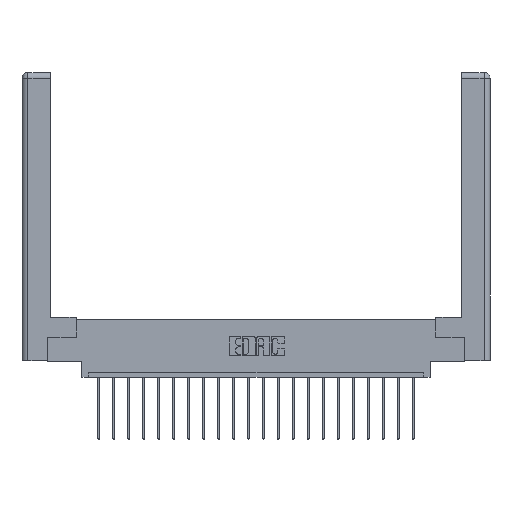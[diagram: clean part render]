
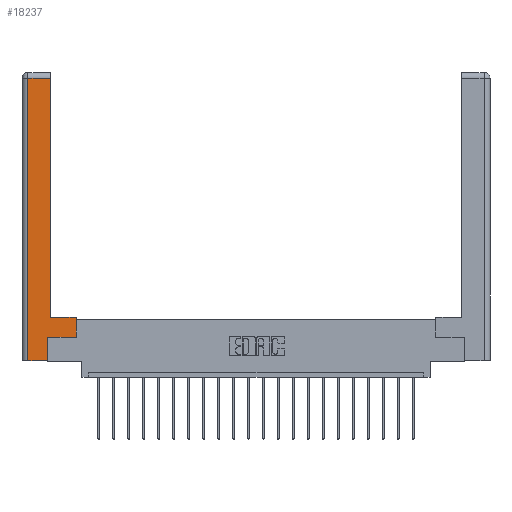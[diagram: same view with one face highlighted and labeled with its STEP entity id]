
A CAD part, top view. The second image highlights one B-rep face of the part: STEP entity #18237.
In plain terms, the highlighted planar face has unit normal (0, 0, 1).
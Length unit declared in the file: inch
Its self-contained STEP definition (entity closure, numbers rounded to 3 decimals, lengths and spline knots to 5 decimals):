
#123 = ORIENTED_EDGE ( 'NONE', *, *, #9968, .T. ) ;
#408 = DIRECTION ( 'NONE',  ( 1., 0., 0. ) ) ;
#514 = ORIENTED_EDGE ( 'NONE', *, *, #17847, .T. ) ;
#659 = VERTEX_POINT ( 'NONE', #21125 ) ;
#902 = ORIENTED_EDGE ( 'NONE', *, *, #16288, .T. ) ;
#1012 = VERTEX_POINT ( 'NONE', #8918 ) ;
#1280 = VECTOR ( 'NONE', #16878, 39.37008 ) ;
#1585 = CARTESIAN_POINT ( 'NONE',  ( 0.0615, 2.94, 0. ) ) ;
#1903 = LINE ( 'NONE', #21490, #8212 ) ;
#2290 = CARTESIAN_POINT ( 'NONE',  ( 0.0615, 2.94, 0. ) ) ;
#2301 = CARTESIAN_POINT ( 'NONE',  ( 0., 0., 0. ) ) ;
#2375 = ORIENTED_EDGE ( 'NONE', *, *, #11505, .T. ) ;
#2445 = ORIENTED_EDGE ( 'NONE', *, *, #6654, .T. ) ;
#2831 = CARTESIAN_POINT ( 'NONE',  ( 0.295, 0.45, 0. ) ) ;
#3074 = DIRECTION ( 'NONE',  ( 0., -1., 0. ) ) ;
#3162 = VERTEX_POINT ( 'NONE', #2831 ) ;
#3676 = VERTEX_POINT ( 'NONE', #1585 ) ;
#3696 = CARTESIAN_POINT ( 'NONE',  ( 0.565, 0.45, 0. ) ) ;
#3892 = VECTOR ( 'NONE', #10589, 39.37008 ) ;
#5469 = LINE ( 'NONE', #3696, #1280 ) ;
#5729 = FACE_OUTER_BOUND ( 'NONE', #6159, .T. ) ;
#5975 = EDGE_CURVE ( 'NONE', #6447, #12346, #18873, .T. ) ;
#6159 = EDGE_LOOP ( 'NONE', ( #123, #2375, #902, #514, #2445, #20924, #20178, #9627 ) ) ;
#6378 = DIRECTION ( 'NONE',  ( -1., 0., 0. ) ) ;
#6447 = VERTEX_POINT ( 'NONE', #14517 ) ;
#6654 = EDGE_CURVE ( 'NONE', #659, #6447, #13541, .T. ) ;
#7048 = DIRECTION ( 'NONE',  ( 0., 1., 0. ) ) ;
#7058 = CARTESIAN_POINT ( 'NONE',  ( 0.565, 0.245, 0. ) ) ;
#7818 = LINE ( 'NONE', #17628, #10714 ) ;
#7833 = LINE ( 'NONE', #2290, #3892 ) ;
#7867 = VECTOR ( 'NONE', #21477, 39.37008 ) ;
#8212 = VECTOR ( 'NONE', #3074, 39.37008 ) ;
#8342 = VECTOR ( 'NONE', #408, 39.37008 ) ;
#8636 = CARTESIAN_POINT ( 'NONE',  ( 0.295, 2.94, 0. ) ) ;
#8918 = CARTESIAN_POINT ( 'NONE',  ( 0.0615, 0., 0. ) ) ;
#9627 = ORIENTED_EDGE ( 'NONE', *, *, #21451, .T. ) ;
#9968 = EDGE_CURVE ( 'NONE', #3162, #17241, #13345, .T. ) ;
#10589 = DIRECTION ( 'NONE',  ( -1., 0., 0. ) ) ;
#10714 = VECTOR ( 'NONE', #6378, 39.37008 ) ;
#10739 = CARTESIAN_POINT ( 'NONE',  ( 0.295, 3., 0. ) ) ;
#10893 = DIRECTION ( 'NONE',  ( -1., 0., 0. ) ) ;
#11313 = EDGE_CURVE ( 'NONE', #12346, #21047, #5469, .T. ) ;
#11505 = EDGE_CURVE ( 'NONE', #17241, #3676, #7833, .T. ) ;
#12336 = PLANE ( 'NONE',  #20123 ) ;
#12346 = VERTEX_POINT ( 'NONE', #17895 ) ;
#13345 = LINE ( 'NONE', #10739, #17835 ) ;
#13541 = LINE ( 'NONE', #14880, #15376 ) ;
#14517 = CARTESIAN_POINT ( 'NONE',  ( 0.265, 0.245, 0. ) ) ;
#14880 = CARTESIAN_POINT ( 'NONE',  ( 0.265, 0.245, 0. ) ) ;
#15376 = VECTOR ( 'NONE', #16559, 39.37008 ) ;
#16288 = EDGE_CURVE ( 'NONE', #3676, #1012, #1903, .T. ) ;
#16559 = DIRECTION ( 'NONE',  ( 0., 1., 0. ) ) ;
#16657 = CARTESIAN_POINT ( 'NONE',  ( 0.565, 0.45, 0. ) ) ;
#16878 = DIRECTION ( 'NONE',  ( 0., 1., 0. ) ) ;
#17241 = VERTEX_POINT ( 'NONE', #8636 ) ;
#17628 = CARTESIAN_POINT ( 'NONE',  ( 0.295, 0.45, 0. ) ) ;
#17835 = VECTOR ( 'NONE', #7048, 39.37008 ) ;
#17847 = EDGE_CURVE ( 'NONE', #1012, #659, #21273, .T. ) ;
#17895 = CARTESIAN_POINT ( 'NONE',  ( 0.565, 0.245, 0. ) ) ;
#18237 = ADVANCED_FACE ( 'NONE', ( #5729 ), #12336, .F. ) ;
#18873 = LINE ( 'NONE', #7058, #8342 ) ;
#19291 = DIRECTION ( 'NONE',  ( 0., 0., -1. ) ) ;
#20123 = AXIS2_PLACEMENT_3D ( 'NONE', #2301, #19291, #10893 ) ;
#20178 = ORIENTED_EDGE ( 'NONE', *, *, #11313, .T. ) ;
#20924 = ORIENTED_EDGE ( 'NONE', *, *, #5975, .T. ) ;
#21047 = VERTEX_POINT ( 'NONE', #16657 ) ;
#21125 = CARTESIAN_POINT ( 'NONE',  ( 0.265, 0., 0. ) ) ;
#21273 = LINE ( 'NONE', #21552, #7867 ) ;
#21451 = EDGE_CURVE ( 'NONE', #21047, #3162, #7818, .T. ) ;
#21477 = DIRECTION ( 'NONE',  ( 1., 0., 0. ) ) ;
#21490 = CARTESIAN_POINT ( 'NONE',  ( 0.0615, 0., 0. ) ) ;
#21552 = CARTESIAN_POINT ( 'NONE',  ( 0.265, 0., 0. ) ) ;
